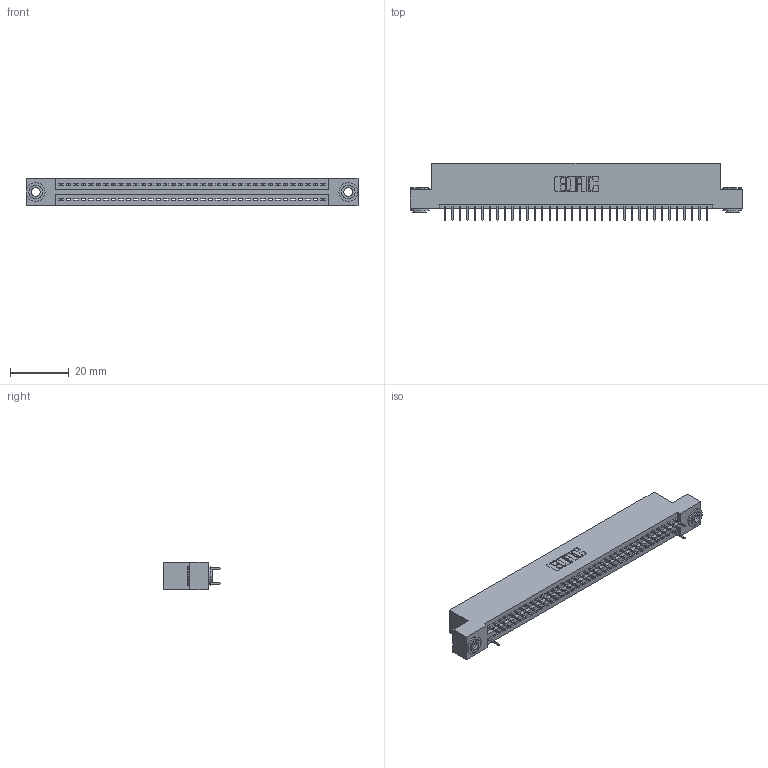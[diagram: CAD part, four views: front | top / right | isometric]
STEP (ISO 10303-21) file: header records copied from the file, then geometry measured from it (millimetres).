
FILE_DESCRIPTION (( 'STEP AP203' ), '1' );
FILE_NAME ('395-072-524-203.STEP', '2018-11-27T10:13:18', ( '' ), ( '' ), 'SwSTEP 2.0', 'SolidWorks 2016', '' );
FILE_SCHEMA (( 'CONFIG_CONTROL_DESIGN' ));
Length unit declared in the file: inch
Products named in the file (4): 345 Part_Flush Mounting Lugs - 0.156 Dia-TH; 395-072-524-203; 345-292-001_345-293-124; 345-250-002_345-250-002-102
Assembly tree (41 placements, depth 2):
  395-072-524-203
    345 Part_Flush Mounting Lugs - 0.156 Dia-TH
    345-292-001_345-293-124  x38
    345-250-002_345-250-002-102  x2
Bounding box: 112.65 x 19.35 x 9.4 mm (x, y, z)
Volume: 10542.6 mm3; surface area: 13784.7 mm2
Topology: 41 solids, 41 shells, 2488 faces, 7149 edges, 4610 vertices
Faces by surface type: plane 1810, cylinder 670, cone 8
Entity records: 28690 total; most frequent: CARTESIAN_POINT 4937, ORIENTED_EDGE 4898, DIRECTION 4355, EDGE_CURVE 2449, LINE 2153, VECTOR 2153, VERTEX_POINT 1626, AXIS2_PLACEMENT_3D 1101
